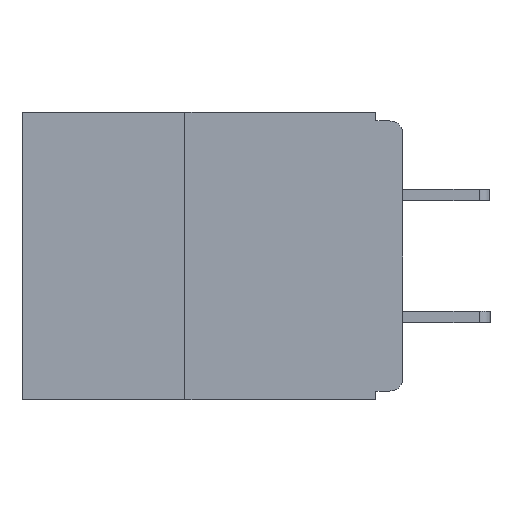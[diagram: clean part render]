
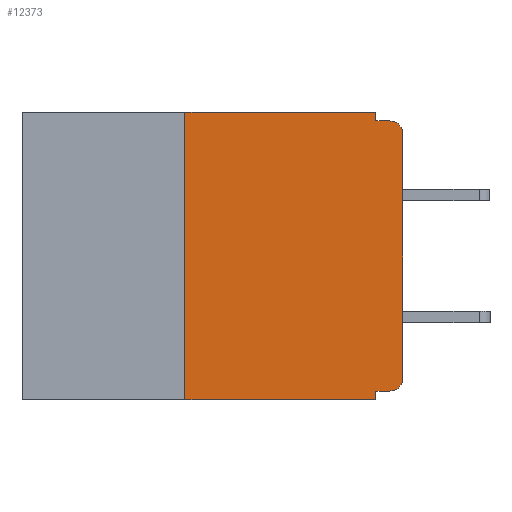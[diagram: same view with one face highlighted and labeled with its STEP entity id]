
A CAD part, left-side view. The second image highlights one B-rep face of the part: STEP entity #12373.
In plain terms, the highlighted planar face has unit normal (-1, 0, 0).
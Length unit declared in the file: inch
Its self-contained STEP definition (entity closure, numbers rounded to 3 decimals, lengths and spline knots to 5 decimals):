
#62 = DIRECTION ( 'NONE',  ( 0., 0., 1. ) ) ;
#290 = CARTESIAN_POINT ( 'NONE',  ( 0., 0.015, -0.32 ) ) ;
#365 = EDGE_CURVE ( 'NONE', #3312, #12075, #3452, .T. ) ;
#390 = VERTEX_POINT ( 'NONE', #7707 ) ;
#573 = LINE ( 'NONE', #16469, #9702 ) ;
#643 = ORIENTED_EDGE ( 'NONE', *, *, #2466, .F. ) ;
#676 = LINE ( 'NONE', #6003, #17339 ) ;
#764 = AXIS2_PLACEMENT_3D ( 'NONE', #5949, #17243, #7569 ) ;
#993 = EDGE_CURVE ( 'NONE', #390, #12877, #17049, .T. ) ;
#1062 = CARTESIAN_POINT ( 'NONE',  ( 0., 0., -0.025 ) ) ;
#1849 = LINE ( 'NONE', #15058, #2359 ) ;
#1883 = CARTESIAN_POINT ( 'NONE',  ( 0., 0.031, -0.01 ) ) ;
#2359 = VECTOR ( 'NONE', #19703, 39.37008 ) ;
#2375 = ORIENTED_EDGE ( 'NONE', *, *, #13605, .F. ) ;
#2466 = EDGE_CURVE ( 'NONE', #14383, #12087, #6999, .T. ) ;
#3312 = VERTEX_POINT ( 'NONE', #5694 ) ;
#3349 = CARTESIAN_POINT ( 'NONE',  ( 0., 0.25, -0.33 ) ) ;
#3452 = LINE ( 'NONE', #3349, #15855 ) ;
#4088 = LINE ( 'NONE', #19358, #7311 ) ;
#4209 = VECTOR ( 'NONE', #6206, 39.37008 ) ;
#4570 = CARTESIAN_POINT ( 'NONE',  ( 0., 0.015, -0.025 ) ) ;
#5144 = CARTESIAN_POINT ( 'NONE',  ( 0., 0.437, 0. ) ) ;
#5331 = AXIS2_PLACEMENT_3D ( 'NONE', #5144, #16446, #6742 ) ;
#5694 = CARTESIAN_POINT ( 'NONE',  ( 0., 0.25, -0.33 ) ) ;
#5739 = CARTESIAN_POINT ( 'NONE',  ( 0., 0.031, 0. ) ) ;
#5949 = CARTESIAN_POINT ( 'NONE',  ( 0., 0.015, -0.305 ) ) ;
#6003 = CARTESIAN_POINT ( 'NONE',  ( 0., 0.437, -0.33 ) ) ;
#6132 = DIRECTION ( 'NONE',  ( 0., 0., -1. ) ) ;
#6206 = DIRECTION ( 'NONE',  ( 0., 0., -1. ) ) ;
#6742 = DIRECTION ( 'NONE',  ( 0., 0., -1. ) ) ;
#6970 = ORIENTED_EDGE ( 'NONE', *, *, #20525, .T. ) ;
#6999 = LINE ( 'NONE', #15373, #18831 ) ;
#7311 = VECTOR ( 'NONE', #62, 39.37008 ) ;
#7350 = VERTEX_POINT ( 'NONE', #290 ) ;
#7569 = DIRECTION ( 'NONE',  ( 0., 0., -1. ) ) ;
#7653 = CARTESIAN_POINT ( 'NONE',  ( 0., 0., -0.305 ) ) ;
#7707 = CARTESIAN_POINT ( 'NONE',  ( 0., 0.031, 0. ) ) ;
#8411 = DIRECTION ( 'NONE',  ( 0., -1., 0. ) ) ;
#8553 = EDGE_LOOP ( 'NONE', ( #17778, #17844, #18040, #18097, #19078, #19644, #20300, #643, #2375, #6970 ) ) ;
#8760 = VERTEX_POINT ( 'NONE', #9153 ) ;
#8830 = EDGE_CURVE ( 'NONE', #3312, #12087, #676, .T. ) ;
#8851 = EDGE_CURVE ( 'NONE', #10689, #8760, #13115, .T. ) ;
#9153 = CARTESIAN_POINT ( 'NONE',  ( 0., 0.015, -0.01 ) ) ;
#9702 = VECTOR ( 'NONE', #8411, 39.37008 ) ;
#10023 = CIRCLE ( 'NONE', #764, 0.015 ) ;
#10431 = CARTESIAN_POINT ( 'NONE',  ( 0., 0.031, -0.32 ) ) ;
#10569 = VECTOR ( 'NONE', #18133, 39.37008 ) ;
#10689 = VERTEX_POINT ( 'NONE', #1062 ) ;
#10897 = DIRECTION ( 'NONE',  ( 0., -1., 0. ) ) ;
#11043 = EDGE_CURVE ( 'NONE', #12075, #390, #573, .T. ) ;
#11089 = LINE ( 'NONE', #16622, #10569 ) ;
#11252 = AXIS2_PLACEMENT_3D ( 'NONE', #4570, #15871, #6132 ) ;
#12075 = VERTEX_POINT ( 'NONE', #15779 ) ;
#12087 = VERTEX_POINT ( 'NONE', #20462 ) ;
#12373 = ADVANCED_FACE ( 'NONE', ( #14289 ), #13236, .F. ) ;
#12877 = VERTEX_POINT ( 'NONE', #1883 ) ;
#13115 = CIRCLE ( 'NONE', #11252, 0.015 ) ;
#13236 = PLANE ( 'NONE',  #5331 ) ;
#13449 = EDGE_CURVE ( 'NONE', #18651, #10689, #4088, .T. ) ;
#13605 = EDGE_CURVE ( 'NONE', #7350, #14383, #1849, .T. ) ;
#14289 = FACE_OUTER_BOUND ( 'NONE', #8553, .T. ) ;
#14383 = VERTEX_POINT ( 'NONE', #10431 ) ;
#15058 = CARTESIAN_POINT ( 'NONE',  ( 0., 0., -0.32 ) ) ;
#15204 = DIRECTION ( 'NONE',  ( 0., 0., -1. ) ) ;
#15373 = CARTESIAN_POINT ( 'NONE',  ( 0., 0.031, -0.33 ) ) ;
#15779 = CARTESIAN_POINT ( 'NONE',  ( 0., 0.25, 0. ) ) ;
#15855 = VECTOR ( 'NONE', #16569, 39.37008 ) ;
#15871 = DIRECTION ( 'NONE',  ( -1., 0., 0. ) ) ;
#16446 = DIRECTION ( 'NONE',  ( 1., 0., 0. ) ) ;
#16452 = EDGE_CURVE ( 'NONE', #12877, #8760, #11089, .T. ) ;
#16469 = CARTESIAN_POINT ( 'NONE',  ( 0., 0.437, 0. ) ) ;
#16569 = DIRECTION ( 'NONE',  ( 0., 0., 1. ) ) ;
#16622 = CARTESIAN_POINT ( 'NONE',  ( 0., 0., -0.01 ) ) ;
#17049 = LINE ( 'NONE', #5739, #4209 ) ;
#17243 = DIRECTION ( 'NONE',  ( -1., 0., 0. ) ) ;
#17339 = VECTOR ( 'NONE', #10897, 39.37008 ) ;
#17778 = ORIENTED_EDGE ( 'NONE', *, *, #13449, .T. ) ;
#17844 = ORIENTED_EDGE ( 'NONE', *, *, #8851, .T. ) ;
#18040 = ORIENTED_EDGE ( 'NONE', *, *, #16452, .F. ) ;
#18097 = ORIENTED_EDGE ( 'NONE', *, *, #993, .F. ) ;
#18133 = DIRECTION ( 'NONE',  ( 0., -1., 0. ) ) ;
#18651 = VERTEX_POINT ( 'NONE', #7653 ) ;
#18831 = VECTOR ( 'NONE', #15204, 39.37008 ) ;
#19078 = ORIENTED_EDGE ( 'NONE', *, *, #11043, .F. ) ;
#19358 = CARTESIAN_POINT ( 'NONE',  ( 0., 0., 0. ) ) ;
#19644 = ORIENTED_EDGE ( 'NONE', *, *, #365, .F. ) ;
#19703 = DIRECTION ( 'NONE',  ( 0., 1., 0. ) ) ;
#20300 = ORIENTED_EDGE ( 'NONE', *, *, #8830, .T. ) ;
#20462 = CARTESIAN_POINT ( 'NONE',  ( 0., 0.031, -0.33 ) ) ;
#20525 = EDGE_CURVE ( 'NONE', #7350, #18651, #10023, .T. ) ;
